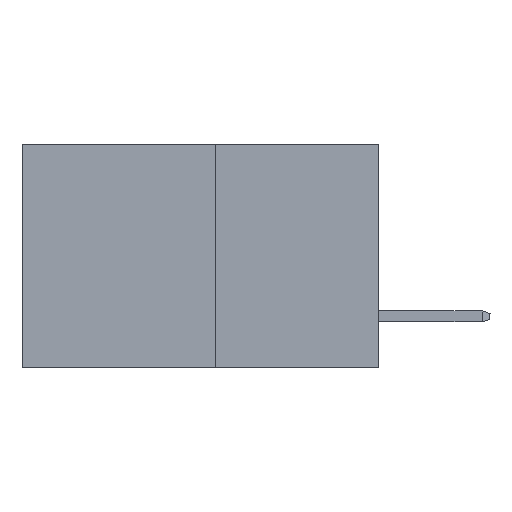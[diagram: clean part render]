
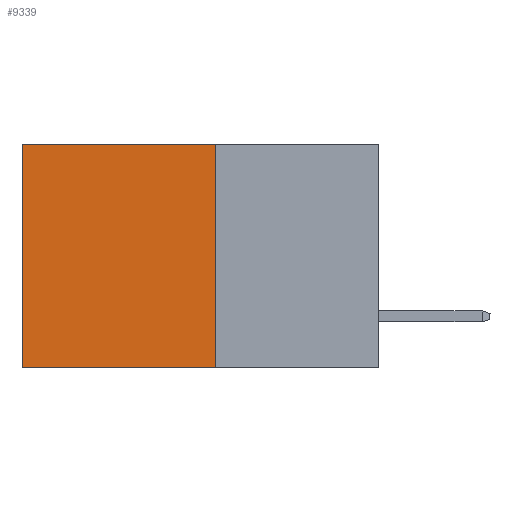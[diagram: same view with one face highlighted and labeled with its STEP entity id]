
A CAD part, left-side view. The second image highlights one B-rep face of the part: STEP entity #9339.
In plain terms, the highlighted planar face has unit normal (-1, 0, 0).
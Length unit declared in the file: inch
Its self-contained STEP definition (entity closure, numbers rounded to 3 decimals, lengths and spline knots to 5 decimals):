
#49 = CARTESIAN_POINT ( 'NONE',  ( 0.277, 0.27, -0.37 ) ) ;
#218 = LINE ( 'NONE', #3512, #4277 ) ;
#276 = LINE ( 'NONE', #828, #6505 ) ;
#520 = DIRECTION ( 'NONE',  ( 0., 0., -1. ) ) ;
#772 = EDGE_CURVE ( 'NONE', #1715, #8293, #6776, .T. ) ;
#828 = CARTESIAN_POINT ( 'NONE',  ( 0.277, 0.59, -0.37 ) ) ;
#1257 = CARTESIAN_POINT ( 'NONE',  ( 0.277, 0.27, -0.37 ) ) ;
#1404 = AXIS2_PLACEMENT_3D ( 'NONE', #4035, #7273, #2418 ) ;
#1715 = VERTEX_POINT ( 'NONE', #8678 ) ;
#2400 = VERTEX_POINT ( 'NONE', #4413 ) ;
#2418 = DIRECTION ( 'NONE',  ( 0., 0., -1. ) ) ;
#3512 = CARTESIAN_POINT ( 'NONE',  ( 0.277, 0.27, 0. ) ) ;
#3563 = EDGE_CURVE ( 'NONE', #2400, #8293, #276, .T. ) ;
#3850 = VECTOR ( 'NONE', #6670, 39.37008 ) ;
#4035 = CARTESIAN_POINT ( 'NONE',  ( 0.277, 0.27, -0.37 ) ) ;
#4277 = VECTOR ( 'NONE', #5143, 39.37008 ) ;
#4413 = CARTESIAN_POINT ( 'NONE',  ( 0.277, 0.59, 0. ) ) ;
#5143 = DIRECTION ( 'NONE',  ( 0., 1., 0. ) ) ;
#5302 = VERTEX_POINT ( 'NONE', #5733 ) ;
#5701 = ORIENTED_EDGE ( 'NONE', *, *, #772, .F. ) ;
#5733 = CARTESIAN_POINT ( 'NONE',  ( 0.277, 0.27, 0. ) ) ;
#6489 = PLANE ( 'NONE',  #1404 ) ;
#6505 = VECTOR ( 'NONE', #520, 39.37008 ) ;
#6621 = ORIENTED_EDGE ( 'NONE', *, *, #3563, .T. ) ;
#6670 = DIRECTION ( 'NONE',  ( 0., 1., 0. ) ) ;
#6763 = DIRECTION ( 'NONE',  ( 0., 0., -1. ) ) ;
#6776 = LINE ( 'NONE', #49, #3850 ) ;
#7273 = DIRECTION ( 'NONE',  ( 1., 0., 0. ) ) ;
#7492 = ORIENTED_EDGE ( 'NONE', *, *, #9096, .T. ) ;
#7881 = FACE_OUTER_BOUND ( 'NONE', #7889, .T. ) ;
#7889 = EDGE_LOOP ( 'NONE', ( #6621, #5701, #10219, #7492 ) ) ;
#8256 = LINE ( 'NONE', #1257, #9999 ) ;
#8293 = VERTEX_POINT ( 'NONE', #9534 ) ;
#8678 = CARTESIAN_POINT ( 'NONE',  ( 0.277, 0.27, -0.37 ) ) ;
#9096 = EDGE_CURVE ( 'NONE', #5302, #2400, #218, .T. ) ;
#9114 = EDGE_CURVE ( 'NONE', #5302, #1715, #8256, .T. ) ;
#9339 = ADVANCED_FACE ( 'NONE', ( #7881 ), #6489, .F. ) ;
#9534 = CARTESIAN_POINT ( 'NONE',  ( 0.277, 0.59, -0.37 ) ) ;
#9999 = VECTOR ( 'NONE', #6763, 39.37008 ) ;
#10219 = ORIENTED_EDGE ( 'NONE', *, *, #9114, .F. ) ;
